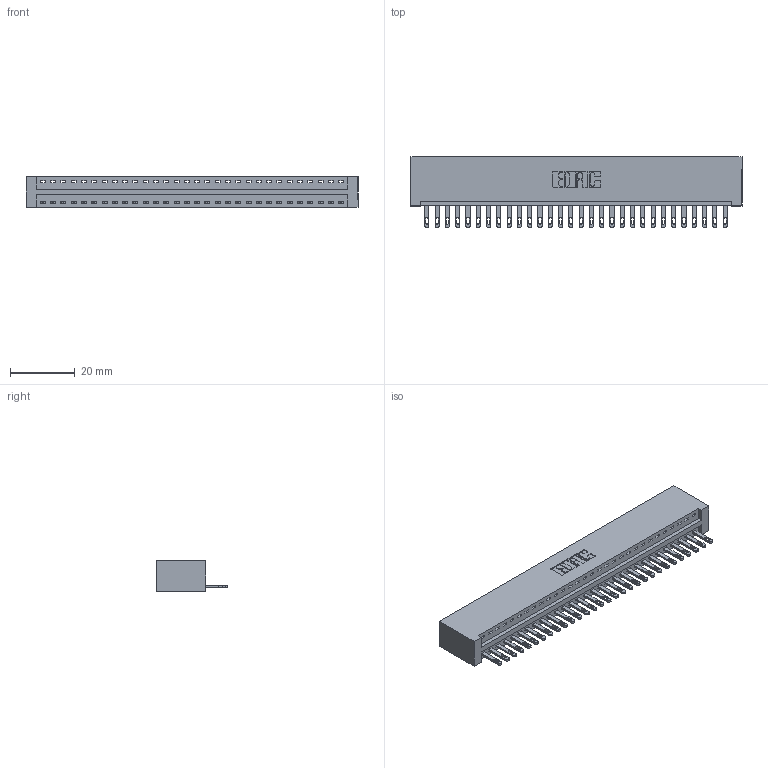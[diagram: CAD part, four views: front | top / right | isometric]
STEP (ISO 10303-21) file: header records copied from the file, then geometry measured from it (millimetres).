
FILE_DESCRIPTION (( 'STEP AP203' ), '1' );
FILE_NAME ('346-030-500-101.STEP', '2018-08-22T03:56:53', ( '' ), ( '' ), 'SwSTEP 2.0', 'SolidWorks 2016', '' );
FILE_SCHEMA (( 'CONFIG_CONTROL_DESIGN' ));
Length unit declared in the file: inch
Products named in the file (3): 346 Part_No Mounting Lugs; 345-292-001_345-293-100; 346-030-500-101
Assembly tree (31 placements, depth 2):
  346-030-500-101
    346 Part_No Mounting Lugs
    345-292-001_345-293-100  x30
Bounding box: 102.49 x 21.84 x 9.4 mm (x, y, z)
Volume: 10295.8 mm3; surface area: 12883.9 mm2
Topology: 31 solids, 31 shells, 1734 faces, 5345 edges, 3562 vertices
Faces by surface type: plane 1092, cylinder 642
Entity records: 19887 total; most frequent: CARTESIAN_POINT 3418, ORIENTED_EDGE 3382, DIRECTION 3027, EDGE_CURVE 1691, LINE 1443, VECTOR 1443, VERTEX_POINT 1126, AXIS2_PLACEMENT_3D 792
